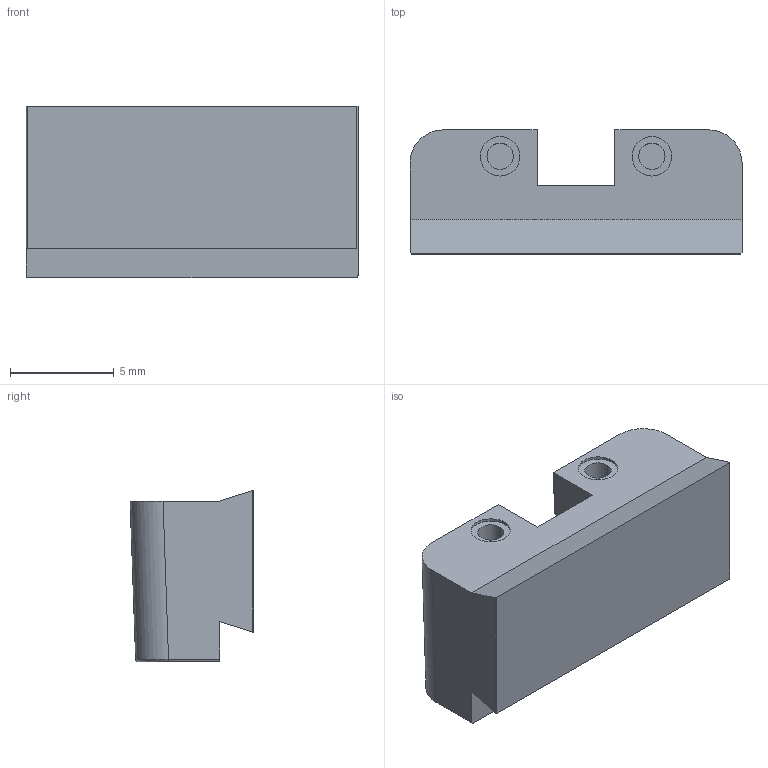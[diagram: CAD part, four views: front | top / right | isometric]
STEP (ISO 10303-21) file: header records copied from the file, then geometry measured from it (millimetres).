
FILE_DESCRIPTION (( 'STEP AP214' ), '1' );
FILE_NAME ('SIGHTS - TRIJICON REAR.STEP', '2013-06-19T14:00:06', ( 'Asher' ), ( '' ), 'SwSTEP 2.0', 'SolidWorks 2013', '' );
FILE_SCHEMA (( 'AUTOMOTIVE_DESIGN' ));
Length unit declared in the file: millimetre
Products named in the file (1): SIGHTS - TRIJICON REAR
Bounding box: 16 x 5.97 x 8.28 mm (x, y, z)
Volume: 579.3 mm3; surface area: 572.1 mm2
Topology: 1 solids, 1 shells, 40 faces, 98 edges, 64 vertices
Faces by surface type: plane 22, cylinder 16, bspline 2
Entity records: 1262 total; most frequent: CARTESIAN_POINT 285, ORIENTED_EDGE 196, DIRECTION 196, EDGE_CURVE 98, AXIS2_PLACEMENT_3D 67, VERTEX_POINT 64, LINE 62, VECTOR 62
